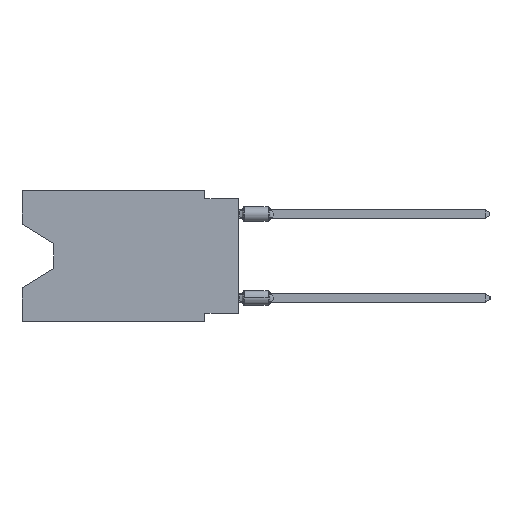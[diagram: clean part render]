
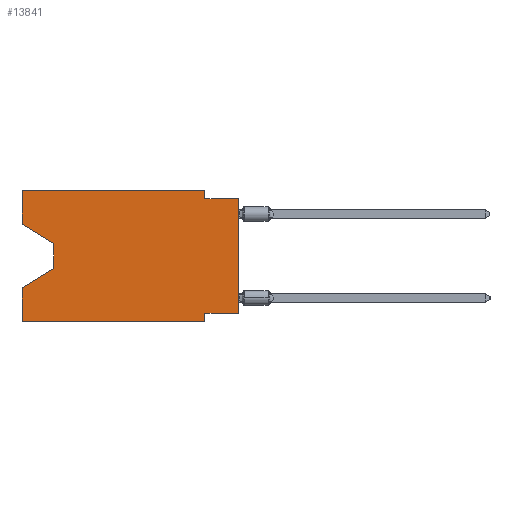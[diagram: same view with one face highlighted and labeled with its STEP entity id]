
A CAD part, left-side view. The second image highlights one B-rep face of the part: STEP entity #13841.
In plain terms, the highlighted planar face has unit normal (-1, 0, 0).
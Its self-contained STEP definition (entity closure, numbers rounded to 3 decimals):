
#191 = VERTEX_POINT ( 'NONE', #39643 ) ;
#537 = EDGE_CURVE ( 'NONE', #32699, #31451, #57704, .T. ) ;
#633 = VECTOR ( 'NONE', #32041, 1000. ) ;
#851 = CARTESIAN_POINT ( 'NONE',  ( 0., 13.97, -5.893 ) ) ;
#1255 = CARTESIAN_POINT ( 'NONE',  ( 0., 13.97, -4.013 ) ) ;
#2556 = CARTESIAN_POINT ( 'NONE',  ( 0., 16.383, 0. ) ) ;
#2941 = CARTESIAN_POINT ( 'NONE',  ( 0., 16.383, -7.36 ) ) ;
#3473 = VECTOR ( 'NONE', #48770, 1000. ) ;
#3504 = EDGE_CURVE ( 'NONE', #191, #60557, #9357, .T. ) ;
#4859 = LINE ( 'NONE', #851, #49171 ) ;
#5166 = DIRECTION ( 'NONE',  ( 0., -1., 0. ) ) ;
#5869 = CARTESIAN_POINT ( 'NONE',  ( 0., 16.383, 0. ) ) ;
#6855 = ORIENTED_EDGE ( 'NONE', *, *, #48684, .F. ) ;
#7475 = LINE ( 'NONE', #2556, #20168 ) ;
#7785 = CARTESIAN_POINT ( 'NONE',  ( 0., 0., -0.635 ) ) ;
#8525 = CARTESIAN_POINT ( 'NONE',  ( 0., 2.54, -9.906 ) ) ;
#9357 = LINE ( 'NONE', #23458, #633 ) ;
#9485 = LINE ( 'NONE', #24791, #56406 ) ;
#10131 = CARTESIAN_POINT ( 'NONE',  ( 0., 16.383, 0. ) ) ;
#10805 = ORIENTED_EDGE ( 'NONE', *, *, #55631, .T. ) ;
#12280 = VERTEX_POINT ( 'NONE', #34151 ) ;
#13126 = VECTOR ( 'NONE', #33637, 1000. ) ;
#13566 = ORIENTED_EDGE ( 'NONE', *, *, #13931, .T. ) ;
#13841 = ADVANCED_FACE ( 'NONE', ( #15679 ), #52768, .F. ) ;
#13931 = EDGE_CURVE ( 'NONE', #50974, #41421, #34961, .T. ) ;
#14067 = CARTESIAN_POINT ( 'NONE',  ( 0., 2.54, -0.635 ) ) ;
#14235 = EDGE_CURVE ( 'NONE', #27662, #31451, #9485, .T. ) ;
#14943 = LINE ( 'NONE', #47434, #13126 ) ;
#14959 = DIRECTION ( 'NONE',  ( 0., 0., 1. ) ) ;
#15679 = FACE_OUTER_BOUND ( 'NONE', #31709, .T. ) ;
#18652 = DIRECTION ( 'NONE',  ( 0., 0., -1. ) ) ;
#19560 = DIRECTION ( 'NONE',  ( 0., 0.855, -0.519 ) ) ;
#19591 = DIRECTION ( 'NONE',  ( 0., -1., 0. ) ) ;
#19731 = VECTOR ( 'NONE', #18652, 1000. ) ;
#20168 = VECTOR ( 'NONE', #14959, 1000. ) ;
#20338 = ORIENTED_EDGE ( 'NONE', *, *, #25266, .F. ) ;
#22480 = LINE ( 'NONE', #60507, #27486 ) ;
#22511 = LINE ( 'NONE', #42136, #59077 ) ;
#22797 = CARTESIAN_POINT ( 'NONE',  ( 0., 13.97, -5.893 ) ) ;
#23458 = CARTESIAN_POINT ( 'NONE',  ( 0., 16.383, -2.546 ) ) ;
#23692 = ORIENTED_EDGE ( 'NONE', *, *, #537, .T. ) ;
#23724 = VECTOR ( 'NONE', #48802, 1000. ) ;
#24791 = CARTESIAN_POINT ( 'NONE',  ( 0., 0., -0.635 ) ) ;
#25266 = EDGE_CURVE ( 'NONE', #36613, #12280, #33667, .T. ) ;
#26062 = CARTESIAN_POINT ( 'NONE',  ( 0., 16.383, -9.906 ) ) ;
#26116 = VECTOR ( 'NONE', #52435, 1000. ) ;
#27186 = VERTEX_POINT ( 'NONE', #22797 ) ;
#27486 = VECTOR ( 'NONE', #42395, 1000. ) ;
#27662 = VERTEX_POINT ( 'NONE', #14067 ) ;
#27929 = ORIENTED_EDGE ( 'NONE', *, *, #3504, .T. ) ;
#28828 = LINE ( 'NONE', #10131, #26116 ) ;
#29842 = ORIENTED_EDGE ( 'NONE', *, *, #59643, .F. ) ;
#30264 = CARTESIAN_POINT ( 'NONE',  ( 0., 2.54, -9.271 ) ) ;
#31451 = VERTEX_POINT ( 'NONE', #7785 ) ;
#31611 = EDGE_CURVE ( 'NONE', #44122, #41421, #22480, .T. ) ;
#31709 = EDGE_LOOP ( 'NONE', ( #27929, #10805, #48482, #6855, #13566, #56830, #44880, #23692, #35919, #29842, #20338, #54206 ) ) ;
#32041 = DIRECTION ( 'NONE',  ( 0., -0.855, -0.519 ) ) ;
#32699 = VERTEX_POINT ( 'NONE', #53249 ) ;
#33637 = DIRECTION ( 'NONE',  ( 0., 1., 0. ) ) ;
#33667 = LINE ( 'NONE', #57266, #44717 ) ;
#33760 = EDGE_CURVE ( 'NONE', #27186, #47473, #4859, .T. ) ;
#34151 = CARTESIAN_POINT ( 'NONE',  ( 0., 2.54, 0. ) ) ;
#34961 = LINE ( 'NONE', #26062, #3473 ) ;
#35919 = ORIENTED_EDGE ( 'NONE', *, *, #14235, .F. ) ;
#36138 = CARTESIAN_POINT ( 'NONE',  ( 0., 16.383, -9.906 ) ) ;
#36613 = VERTEX_POINT ( 'NONE', #5869 ) ;
#36909 = DIRECTION ( 'NONE',  ( 0., 0., -1. ) ) ;
#38960 = DIRECTION ( 'NONE',  ( 0., 0., -1. ) ) ;
#39643 = CARTESIAN_POINT ( 'NONE',  ( 0., 16.383, -2.546 ) ) ;
#41421 = VERTEX_POINT ( 'NONE', #8525 ) ;
#42136 = CARTESIAN_POINT ( 'NONE',  ( 0., 2.54, 0. ) ) ;
#42395 = DIRECTION ( 'NONE',  ( 0., 0., -1. ) ) ;
#42653 = CARTESIAN_POINT ( 'NONE',  ( 0., 16.383, 0. ) ) ;
#42965 = DIRECTION ( 'NONE',  ( 1., 0., 0. ) ) ;
#44122 = VERTEX_POINT ( 'NONE', #30264 ) ;
#44717 = VECTOR ( 'NONE', #5166, 1000. ) ;
#44880 = ORIENTED_EDGE ( 'NONE', *, *, #46154, .F. ) ;
#45639 = CARTESIAN_POINT ( 'NONE',  ( 0., 0., 0. ) ) ;
#46154 = EDGE_CURVE ( 'NONE', #32699, #44122, #14943, .T. ) ;
#46560 = AXIS2_PLACEMENT_3D ( 'NONE', #42653, #42965, #38960 ) ;
#47434 = CARTESIAN_POINT ( 'NONE',  ( 0., 0., -9.271 ) ) ;
#47473 = VERTEX_POINT ( 'NONE', #2941 ) ;
#48482 = ORIENTED_EDGE ( 'NONE', *, *, #33760, .T. ) ;
#48684 = EDGE_CURVE ( 'NONE', #50974, #47473, #7475, .T. ) ;
#48770 = DIRECTION ( 'NONE',  ( 0., -1., 0. ) ) ;
#48802 = DIRECTION ( 'NONE',  ( 0., 0., 1. ) ) ;
#49171 = VECTOR ( 'NONE', #19560, 1000. ) ;
#49352 = EDGE_CURVE ( 'NONE', #191, #36613, #28828, .T. ) ;
#50974 = VERTEX_POINT ( 'NONE', #36138 ) ;
#52435 = DIRECTION ( 'NONE',  ( 0., 0., 1. ) ) ;
#52768 = PLANE ( 'NONE',  #46560 ) ;
#53249 = CARTESIAN_POINT ( 'NONE',  ( 0., 0., -9.271 ) ) ;
#54206 = ORIENTED_EDGE ( 'NONE', *, *, #49352, .F. ) ;
#55631 = EDGE_CURVE ( 'NONE', #60557, #27186, #59147, .T. ) ;
#56406 = VECTOR ( 'NONE', #19591, 1000. ) ;
#56830 = ORIENTED_EDGE ( 'NONE', *, *, #31611, .F. ) ;
#56965 = CARTESIAN_POINT ( 'NONE',  ( 0., 13.97, -4.013 ) ) ;
#57266 = CARTESIAN_POINT ( 'NONE',  ( 0., 16.383, 0. ) ) ;
#57704 = LINE ( 'NONE', #45639, #23724 ) ;
#59077 = VECTOR ( 'NONE', #36909, 1000. ) ;
#59147 = LINE ( 'NONE', #56965, #19731 ) ;
#59643 = EDGE_CURVE ( 'NONE', #12280, #27662, #22511, .T. ) ;
#60507 = CARTESIAN_POINT ( 'NONE',  ( 0., 2.54, -9.906 ) ) ;
#60557 = VERTEX_POINT ( 'NONE', #1255 ) ;
